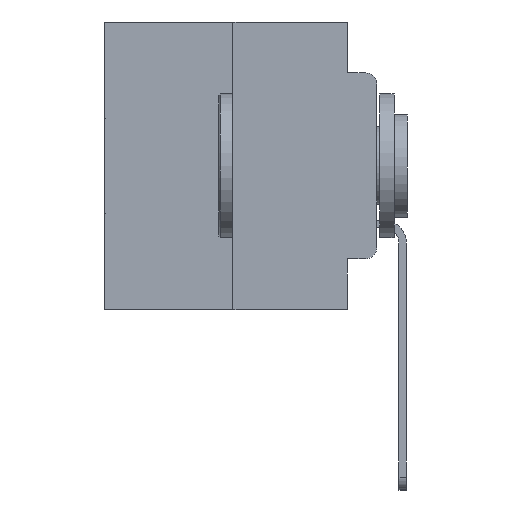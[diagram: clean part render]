
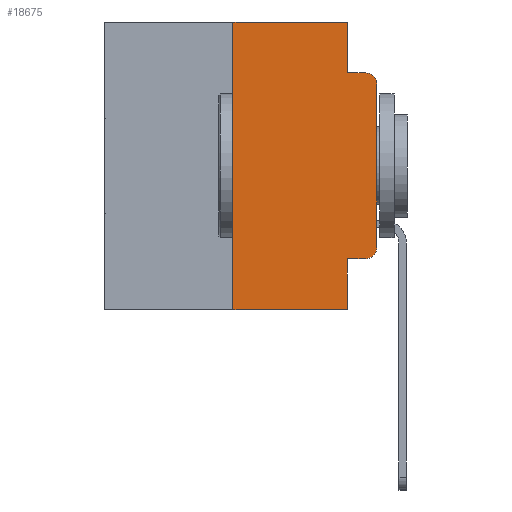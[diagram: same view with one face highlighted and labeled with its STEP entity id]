
A CAD part, left-side view. The second image highlights one B-rep face of the part: STEP entity #18675.
In plain terms, the highlighted planar face has unit normal (-1, 0, 0).
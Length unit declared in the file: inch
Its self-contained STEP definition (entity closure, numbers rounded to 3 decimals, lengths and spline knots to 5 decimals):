
#30 = CARTESIAN_POINT ( 'NONE',  ( 0., 0.473, 0. ) ) ;
#640 = VERTEX_POINT ( 'NONE', #14555 ) ;
#735 = CARTESIAN_POINT ( 'NONE',  ( 0., 0.051, 0. ) ) ;
#906 = CARTESIAN_POINT ( 'NONE',  ( 0., 0.473, -0.5 ) ) ;
#1023 = CARTESIAN_POINT ( 'NONE',  ( 0., 0.051, -0.4115 ) ) ;
#1215 = FACE_OUTER_BOUND ( 'NONE', #5708, .T. ) ;
#1603 = VECTOR ( 'NONE', #4139, 39.37008 ) ;
#2455 = ORIENTED_EDGE ( 'NONE', *, *, #26147, .F. ) ;
#2468 = CARTESIAN_POINT ( 'NONE',  ( 0., 0.051, -0.5 ) ) ;
#2536 = EDGE_CURVE ( 'NONE', #640, #23294, #23727, .T. ) ;
#2776 = VECTOR ( 'NONE', #18120, 39.37008 ) ;
#3081 = CARTESIAN_POINT ( 'NONE',  ( 0., 0.25, -0.5 ) ) ;
#4138 = DIRECTION ( 'NONE',  ( 0., 0., -1. ) ) ;
#4139 = DIRECTION ( 'NONE',  ( 0., 0., 1. ) ) ;
#4167 = DIRECTION ( 'NONE',  ( -1., 0., 0. ) ) ;
#4225 = LINE ( 'NONE', #6877, #2776 ) ;
#4370 = DIRECTION ( 'NONE',  ( 0., 0., 1. ) ) ;
#4594 = CARTESIAN_POINT ( 'NONE',  ( 0., 0.02, -0.1085 ) ) ;
#4877 = PLANE ( 'NONE',  #22042 ) ;
#4974 = DIRECTION ( 'NONE',  ( 0., 0., -1. ) ) ;
#5335 = VERTEX_POINT ( 'NONE', #9106 ) ;
#5668 = CIRCLE ( 'NONE', #21837, 0.02 ) ;
#5708 = EDGE_LOOP ( 'NONE', ( #20031, #8869, #26597, #6406, #7109, #19006, #13768, #2455, #9233, #9966 ) ) ;
#6406 = ORIENTED_EDGE ( 'NONE', *, *, #13693, .F. ) ;
#6431 = CARTESIAN_POINT ( 'NONE',  ( 0., 0.25, 0. ) ) ;
#6767 = CARTESIAN_POINT ( 'NONE',  ( 0., 0.02, -0.3915 ) ) ;
#6787 = AXIS2_PLACEMENT_3D ( 'NONE', #4594, #4167, #4138 ) ;
#6815 = VERTEX_POINT ( 'NONE', #26643 ) ;
#6845 = CARTESIAN_POINT ( 'NONE',  ( 0., 0.051, 0. ) ) ;
#6877 = CARTESIAN_POINT ( 'NONE',  ( 0., 0.473, 0. ) ) ;
#7109 = ORIENTED_EDGE ( 'NONE', *, *, #17333, .F. ) ;
#7736 = DIRECTION ( 'NONE',  ( 0., -1., 0. ) ) ;
#8285 = LINE ( 'NONE', #906, #19463 ) ;
#8658 = EDGE_CURVE ( 'NONE', #13280, #640, #12683, .T. ) ;
#8869 = ORIENTED_EDGE ( 'NONE', *, *, #2536, .T. ) ;
#8903 = VECTOR ( 'NONE', #12306, 39.37008 ) ;
#9046 = DIRECTION ( 'NONE',  ( 0., 0., -1. ) ) ;
#9106 = CARTESIAN_POINT ( 'NONE',  ( 0., 0.25, 0. ) ) ;
#9209 = EDGE_CURVE ( 'NONE', #13297, #5335, #19609, .T. ) ;
#9233 = ORIENTED_EDGE ( 'NONE', *, *, #18749, .T. ) ;
#9283 = LINE ( 'NONE', #6845, #26310 ) ;
#9623 = LINE ( 'NONE', #14546, #8903 ) ;
#9966 = ORIENTED_EDGE ( 'NONE', *, *, #17257, .T. ) ;
#10054 = DIRECTION ( 'NONE',  ( 0., -1., 0. ) ) ;
#11214 = VECTOR ( 'NONE', #27462, 39.37008 ) ;
#11283 = VECTOR ( 'NONE', #4370, 39.37008 ) ;
#11982 = CARTESIAN_POINT ( 'NONE',  ( 0., 0., -0.3915 ) ) ;
#12306 = DIRECTION ( 'NONE',  ( 0., 0., -1. ) ) ;
#12683 = LINE ( 'NONE', #17820, #11283 ) ;
#12749 = LINE ( 'NONE', #21101, #29012 ) ;
#13157 = VERTEX_POINT ( 'NONE', #2468 ) ;
#13280 = VERTEX_POINT ( 'NONE', #11982 ) ;
#13297 = VERTEX_POINT ( 'NONE', #3081 ) ;
#13693 = EDGE_CURVE ( 'NONE', #26065, #17612, #9283, .T. ) ;
#13768 = ORIENTED_EDGE ( 'NONE', *, *, #24875, .T. ) ;
#14546 = CARTESIAN_POINT ( 'NONE',  ( 0., 0.051, 0. ) ) ;
#14555 = CARTESIAN_POINT ( 'NONE',  ( 0., 0., -0.1085 ) ) ;
#14704 = CARTESIAN_POINT ( 'NONE',  ( 0., 0.051, -0.0885 ) ) ;
#16138 = VERTEX_POINT ( 'NONE', #1023 ) ;
#16701 = EDGE_CURVE ( 'NONE', #17612, #23294, #12749, .T. ) ;
#17257 = EDGE_CURVE ( 'NONE', #6815, #13280, #5668, .T. ) ;
#17333 = EDGE_CURVE ( 'NONE', #5335, #26065, #4225, .T. ) ;
#17612 = VERTEX_POINT ( 'NONE', #14704 ) ;
#17820 = CARTESIAN_POINT ( 'NONE',  ( 0., 0., 0. ) ) ;
#17827 = LINE ( 'NONE', #25257, #11214 ) ;
#18120 = DIRECTION ( 'NONE',  ( 0., -1., 0. ) ) ;
#18384 = DIRECTION ( 'NONE',  ( 1., 0., 0. ) ) ;
#18675 = ADVANCED_FACE ( 'NONE', ( #1215 ), #4877, .F. ) ;
#18749 = EDGE_CURVE ( 'NONE', #16138, #6815, #17827, .T. ) ;
#19006 = ORIENTED_EDGE ( 'NONE', *, *, #9209, .F. ) ;
#19463 = VECTOR ( 'NONE', #10054, 39.37008 ) ;
#19609 = LINE ( 'NONE', #6431, #1603 ) ;
#20031 = ORIENTED_EDGE ( 'NONE', *, *, #8658, .T. ) ;
#21101 = CARTESIAN_POINT ( 'NONE',  ( 0., 0.051, -0.0885 ) ) ;
#21837 = AXIS2_PLACEMENT_3D ( 'NONE', #6767, #22370, #9046 ) ;
#22042 = AXIS2_PLACEMENT_3D ( 'NONE', #30, #18384, #4974 ) ;
#22370 = DIRECTION ( 'NONE',  ( -1., 0., 0. ) ) ;
#23294 = VERTEX_POINT ( 'NONE', #23836 ) ;
#23727 = CIRCLE ( 'NONE', #6787, 0.02 ) ;
#23836 = CARTESIAN_POINT ( 'NONE',  ( 0., 0.02, -0.0885 ) ) ;
#24875 = EDGE_CURVE ( 'NONE', #13297, #13157, #8285, .T. ) ;
#25257 = CARTESIAN_POINT ( 'NONE',  ( 0., 0.051, -0.4115 ) ) ;
#26065 = VERTEX_POINT ( 'NONE', #735 ) ;
#26147 = EDGE_CURVE ( 'NONE', #16138, #13157, #9623, .T. ) ;
#26310 = VECTOR ( 'NONE', #26874, 39.37008 ) ;
#26597 = ORIENTED_EDGE ( 'NONE', *, *, #16701, .F. ) ;
#26643 = CARTESIAN_POINT ( 'NONE',  ( 0., 0.02, -0.4115 ) ) ;
#26874 = DIRECTION ( 'NONE',  ( 0., 0., -1. ) ) ;
#27462 = DIRECTION ( 'NONE',  ( 0., -1., 0. ) ) ;
#29012 = VECTOR ( 'NONE', #7736, 39.37008 ) ;
